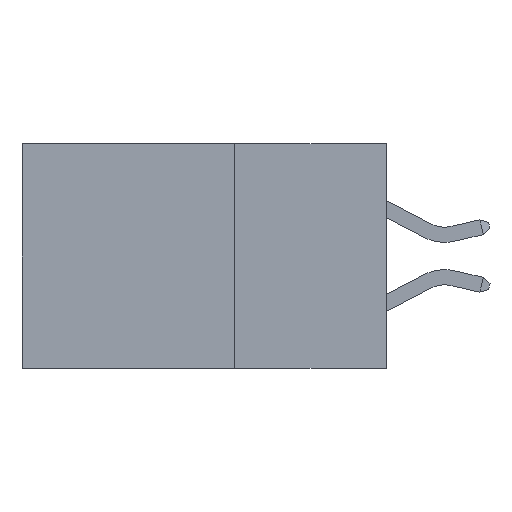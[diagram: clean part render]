
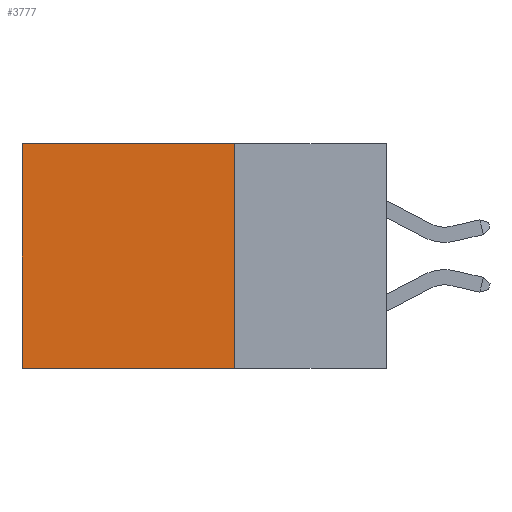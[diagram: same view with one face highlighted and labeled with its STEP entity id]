
A CAD part, left-side view. The second image highlights one B-rep face of the part: STEP entity #3777.
In plain terms, the highlighted planar face has unit normal (-1, 0, 0).
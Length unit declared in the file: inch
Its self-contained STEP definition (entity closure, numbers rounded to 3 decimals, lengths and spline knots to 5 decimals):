
#15 = DIRECTION ( 'NONE',  ( 0., 0., -1. ) ) ;
#1245 = VERTEX_POINT ( 'NONE', #7255 ) ;
#1751 = VECTOR ( 'NONE', #8709, 39.37008 ) ;
#1842 = VECTOR ( 'NONE', #8561, 39.37008 ) ;
#2044 = CARTESIAN_POINT ( 'NONE',  ( 0.2615, 0.25, -0.37 ) ) ;
#2476 = ORIENTED_EDGE ( 'NONE', *, *, #3225, .T. ) ;
#2556 = LINE ( 'NONE', #2044, #6560 ) ;
#3225 = EDGE_CURVE ( 'NONE', #1245, #8045, #9705, .T. ) ;
#3492 = CARTESIAN_POINT ( 'NONE',  ( 0.2615, 0.25, 0. ) ) ;
#3764 = LINE ( 'NONE', #5032, #1751 ) ;
#3777 = ADVANCED_FACE ( 'NONE', ( #5326 ), #9228, .F. ) ;
#4113 = LINE ( 'NONE', #6426, #1842 ) ;
#4233 = ORIENTED_EDGE ( 'NONE', *, *, #6256, .T. ) ;
#4292 = VECTOR ( 'NONE', #9405, 39.37008 ) ;
#4836 = DIRECTION ( 'NONE',  ( 1., 0., 0. ) ) ;
#4976 = CARTESIAN_POINT ( 'NONE',  ( 0.2615, 0.25, -0.37 ) ) ;
#5032 = CARTESIAN_POINT ( 'NONE',  ( 0.2615, 0.6, -0.37 ) ) ;
#5326 = FACE_OUTER_BOUND ( 'NONE', #9285, .T. ) ;
#5412 = CARTESIAN_POINT ( 'NONE',  ( 0.2615, 0.6, 0. ) ) ;
#6256 = EDGE_CURVE ( 'NONE', #8045, #9357, #3764, .T. ) ;
#6426 = CARTESIAN_POINT ( 'NONE',  ( 0.2615, 0.25, -0.37 ) ) ;
#6560 = VECTOR ( 'NONE', #7284, 39.37008 ) ;
#7255 = CARTESIAN_POINT ( 'NONE',  ( 0.2615, 0.25, 0. ) ) ;
#7284 = DIRECTION ( 'NONE',  ( 0., 1., 0. ) ) ;
#7428 = CARTESIAN_POINT ( 'NONE',  ( 0.2615, 0.6, -0.37 ) ) ;
#7506 = EDGE_CURVE ( 'NONE', #1245, #9100, #4113, .T. ) ;
#7748 = CARTESIAN_POINT ( 'NONE',  ( 0.2615, 0.25, -0.37 ) ) ;
#8045 = VERTEX_POINT ( 'NONE', #5412 ) ;
#8561 = DIRECTION ( 'NONE',  ( 0., 0., -1. ) ) ;
#8709 = DIRECTION ( 'NONE',  ( 0., 0., -1. ) ) ;
#8870 = ORIENTED_EDGE ( 'NONE', *, *, #9205, .F. ) ;
#9100 = VERTEX_POINT ( 'NONE', #4976 ) ;
#9126 = AXIS2_PLACEMENT_3D ( 'NONE', #7748, #4836, #15 ) ;
#9169 = ORIENTED_EDGE ( 'NONE', *, *, #7506, .F. ) ;
#9205 = EDGE_CURVE ( 'NONE', #9100, #9357, #2556, .T. ) ;
#9228 = PLANE ( 'NONE',  #9126 ) ;
#9285 = EDGE_LOOP ( 'NONE', ( #4233, #8870, #9169, #2476 ) ) ;
#9357 = VERTEX_POINT ( 'NONE', #7428 ) ;
#9405 = DIRECTION ( 'NONE',  ( 0., 1., 0. ) ) ;
#9705 = LINE ( 'NONE', #3492, #4292 ) ;
